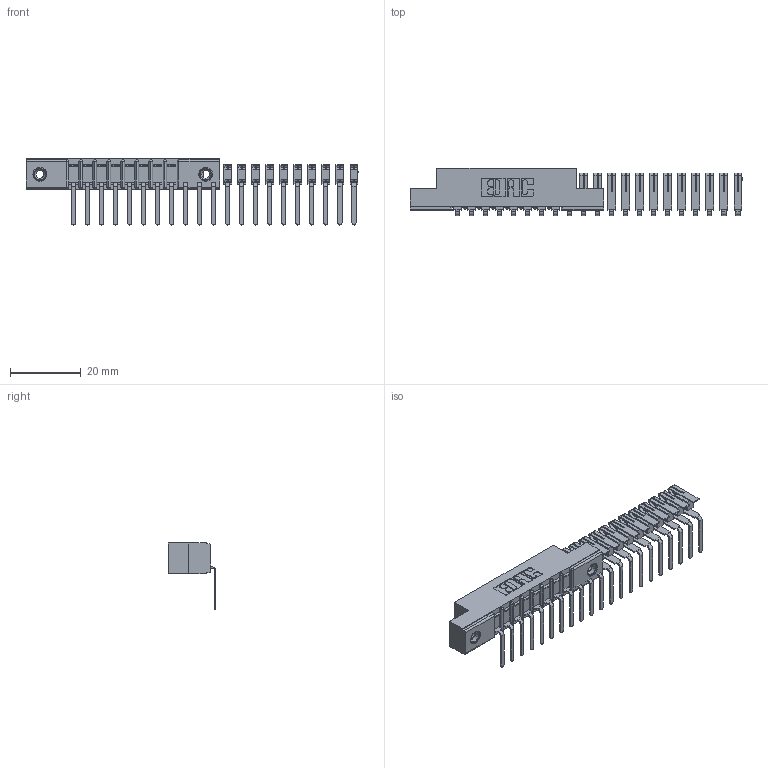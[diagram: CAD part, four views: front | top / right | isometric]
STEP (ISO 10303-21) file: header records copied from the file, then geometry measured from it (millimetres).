
FILE_DESCRIPTION (( 'STEP AP203' ), '1' );
FILE_NAME ('357-021-557-108.STEP', '2018-08-08T21:42:35', ( '' ), ( '' ), 'SwSTEP 2.0', 'SolidWorks 2016', '' );
FILE_SCHEMA (( 'CONFIG_CONTROL_DESIGN' ));
Length unit declared in the file: inch
Products named in the file (4): 307 Part_.156 Dia Mounting Holes; 307-290-002_557; 345-250-001_345-250-003-102; 357-021-557-108
Assembly tree (24 placements, depth 2):
  357-021-557-108
    307 Part_.156 Dia Mounting Holes
    307-290-002_557  x21
    345-250-001_345-250-003-102  x2
Bounding box: 93.87 x 13.32 x 18.67 mm (x, y, z)
Volume: 4031 mm3; surface area: 9110.5 mm2
Topology: 24 solids, 24 shells, 1565 faces, 4751 edges, 3134 vertices
Faces by surface type: plane 933, cylinder 598, sphere 18, cone 12, torus 4
Entity records: 13505 total; most frequent: CARTESIAN_POINT 2196, DIRECTION 2173, ORIENTED_EDGE 2166, EDGE_CURVE 1083, LINE 811, VECTOR 811, VERTEX_POINT 704, AXIS2_PLACEMENT_3D 681
